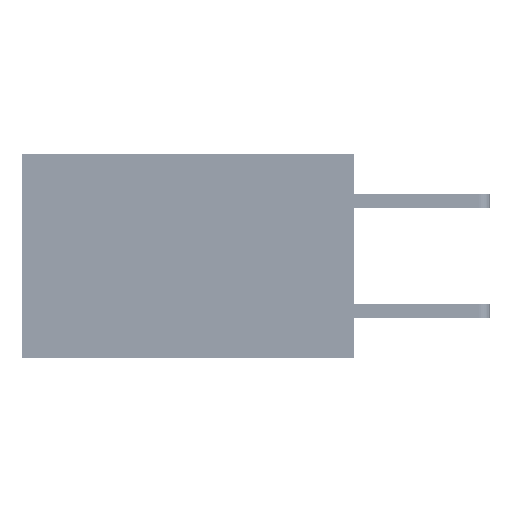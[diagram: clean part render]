
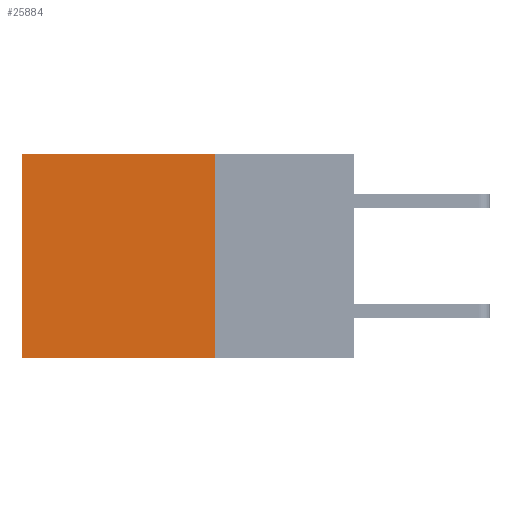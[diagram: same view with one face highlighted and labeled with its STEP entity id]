
A CAD part, left-side view. The second image highlights one B-rep face of the part: STEP entity #25884.
In plain terms, the highlighted planar face has unit normal (-1, 0, 0).
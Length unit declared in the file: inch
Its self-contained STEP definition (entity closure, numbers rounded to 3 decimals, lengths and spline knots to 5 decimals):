
#525 = DIRECTION ( 'NONE',  ( 0., 0., -1. ) ) ;
#2310 = AXIS2_PLACEMENT_3D ( 'NONE', #20770, #33366, #14609 ) ;
#4910 = CARTESIAN_POINT ( 'NONE',  ( 0.2875, 0.25, 0. ) ) ;
#5193 = VECTOR ( 'NONE', #39084, 39.37008 ) ;
#6575 = VECTOR ( 'NONE', #30132, 39.37008 ) ;
#8146 = LINE ( 'NONE', #35752, #16568 ) ;
#8220 = VERTEX_POINT ( 'NONE', #16998 ) ;
#10936 = CARTESIAN_POINT ( 'NONE',  ( 0.2875, 0.25, 0. ) ) ;
#11669 = FACE_OUTER_BOUND ( 'NONE', #38407, .T. ) ;
#14609 = DIRECTION ( 'NONE',  ( 0., 0., -1. ) ) ;
#14933 = CARTESIAN_POINT ( 'NONE',  ( 0.2875, 0.6, 0. ) ) ;
#16568 = VECTOR ( 'NONE', #38904, 39.37008 ) ;
#16998 = CARTESIAN_POINT ( 'NONE',  ( 0.2875, 0.25, -0.37 ) ) ;
#19717 = VERTEX_POINT ( 'NONE', #23526 ) ;
#20503 = LINE ( 'NONE', #35065, #34214 ) ;
#20770 = CARTESIAN_POINT ( 'NONE',  ( 0.2875, 0.25, 0. ) ) ;
#21270 = VERTEX_POINT ( 'NONE', #14933 ) ;
#21690 = EDGE_CURVE ( 'NONE', #38457, #21270, #29733, .T. ) ;
#22267 = ORIENTED_EDGE ( 'NONE', *, *, #32386, .F. ) ;
#23526 = CARTESIAN_POINT ( 'NONE',  ( 0.2875, 0.6, -0.37 ) ) ;
#24707 = ORIENTED_EDGE ( 'NONE', *, *, #36510, .F. ) ;
#25884 = ADVANCED_FACE ( 'NONE', ( #11669 ), #30235, .F. ) ;
#29733 = LINE ( 'NONE', #4910, #6575 ) ;
#30132 = DIRECTION ( 'NONE',  ( 0., 1., 0. ) ) ;
#30235 = PLANE ( 'NONE',  #2310 ) ;
#30341 = LINE ( 'NONE', #35934, #5193 ) ;
#31880 = ORIENTED_EDGE ( 'NONE', *, *, #36087, .T. ) ;
#32386 = EDGE_CURVE ( 'NONE', #38457, #8220, #20503, .T. ) ;
#33366 = DIRECTION ( 'NONE',  ( 1., 0., 0. ) ) ;
#34214 = VECTOR ( 'NONE', #525, 39.37008 ) ;
#35065 = CARTESIAN_POINT ( 'NONE',  ( 0.2875, 0.25, 0. ) ) ;
#35136 = ORIENTED_EDGE ( 'NONE', *, *, #21690, .T. ) ;
#35752 = CARTESIAN_POINT ( 'NONE',  ( 0.2875, 0.25, -0.37 ) ) ;
#35934 = CARTESIAN_POINT ( 'NONE',  ( 0.2875, 0.6, 0. ) ) ;
#36087 = EDGE_CURVE ( 'NONE', #21270, #19717, #30341, .T. ) ;
#36510 = EDGE_CURVE ( 'NONE', #8220, #19717, #8146, .T. ) ;
#38407 = EDGE_LOOP ( 'NONE', ( #31880, #24707, #22267, #35136 ) ) ;
#38457 = VERTEX_POINT ( 'NONE', #10936 ) ;
#38904 = DIRECTION ( 'NONE',  ( 0., 1., 0. ) ) ;
#39084 = DIRECTION ( 'NONE',  ( 0., 0., -1. ) ) ;
